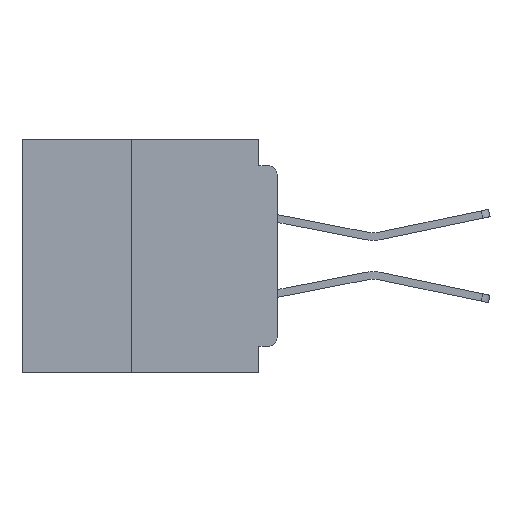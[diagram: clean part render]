
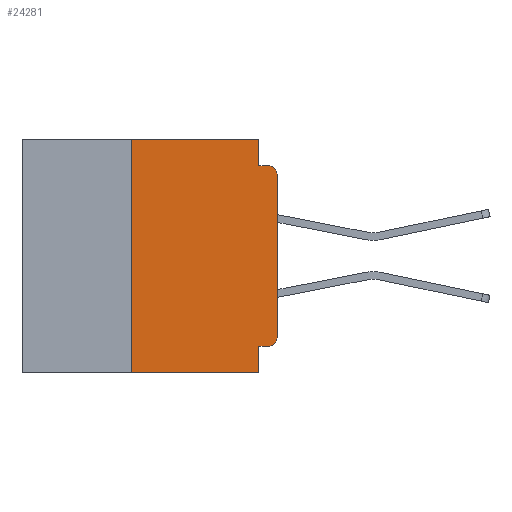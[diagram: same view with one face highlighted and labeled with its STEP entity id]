
A CAD part, left-side view. The second image highlights one B-rep face of the part: STEP entity #24281.
In plain terms, the highlighted planar face has unit normal (-1, 0, 0).
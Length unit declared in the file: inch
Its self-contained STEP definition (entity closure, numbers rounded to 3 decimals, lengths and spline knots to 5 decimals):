
#169 = EDGE_CURVE ( 'NONE', #33190, #14834, #8546, .T. ) ;
#683 = AXIS2_PLACEMENT_3D ( 'NONE', #11805, #33521, #14911 ) ;
#696 = LINE ( 'NONE', #1604, #8038 ) ;
#1527 = DIRECTION ( 'NONE',  ( 0., 0., -1. ) ) ;
#1538 = DIRECTION ( 'NONE',  ( 0., 0., -1. ) ) ;
#1604 = CARTESIAN_POINT ( 'NONE',  ( 0., 0., -0.045 ) ) ;
#1689 = AXIS2_PLACEMENT_3D ( 'NONE', #35556, #29384, #1527 ) ;
#1912 = CARTESIAN_POINT ( 'NONE',  ( 0., 0.031, -0.4 ) ) ;
#3444 = AXIS2_PLACEMENT_3D ( 'NONE', #34811, #16224, #37923 ) ;
#4148 = VERTEX_POINT ( 'NONE', #24754 ) ;
#4276 = VECTOR ( 'NONE', #1538, 39.37008 ) ;
#4750 = LINE ( 'NONE', #22648, #12005 ) ;
#5132 = CARTESIAN_POINT ( 'NONE',  ( 0., 0.031, -0.045 ) ) ;
#5250 = DIRECTION ( 'NONE',  ( 0., -1., 0. ) ) ;
#6891 = CARTESIAN_POINT ( 'NONE',  ( 0., 0.031, -0.355 ) ) ;
#6967 = VERTEX_POINT ( 'NONE', #36861 ) ;
#7402 = CARTESIAN_POINT ( 'NONE',  ( 0., 0.437, 0. ) ) ;
#7459 = EDGE_CURVE ( 'NONE', #32794, #4148, #23890, .T. ) ;
#7644 = CARTESIAN_POINT ( 'NONE',  ( 0., 0.031, 0. ) ) ;
#8038 = VECTOR ( 'NONE', #20191, 39.37008 ) ;
#8229 = ORIENTED_EDGE ( 'NONE', *, *, #169, .T. ) ;
#8308 = ORIENTED_EDGE ( 'NONE', *, *, #9075, .T. ) ;
#8374 = VECTOR ( 'NONE', #29146, 39.37008 ) ;
#8546 = LINE ( 'NONE', #17950, #32329 ) ;
#9075 = EDGE_CURVE ( 'NONE', #14834, #6967, #13033, .T. ) ;
#9210 = ORIENTED_EDGE ( 'NONE', *, *, #35574, .F. ) ;
#9241 = ORIENTED_EDGE ( 'NONE', *, *, #33174, .F. ) ;
#9282 = ORIENTED_EDGE ( 'NONE', *, *, #21765, .F. ) ;
#9529 = EDGE_CURVE ( 'NONE', #21045, #4148, #20307, .T. ) ;
#10096 = CARTESIAN_POINT ( 'NONE',  ( 0., 0.015, -0.355 ) ) ;
#10304 = ORIENTED_EDGE ( 'NONE', *, *, #37301, .F. ) ;
#10667 = ORIENTED_EDGE ( 'NONE', *, *, #7459, .T. ) ;
#10715 = VERTEX_POINT ( 'NONE', #35857 ) ;
#11273 = DIRECTION ( 'NONE',  ( 0., 0., -1. ) ) ;
#11653 = ORIENTED_EDGE ( 'NONE', *, *, #9529, .F. ) ;
#11805 = CARTESIAN_POINT ( 'NONE',  ( 0., 0.015, -0.34 ) ) ;
#12005 = VECTOR ( 'NONE', #25786, 39.37008 ) ;
#12025 = VECTOR ( 'NONE', #11273, 39.37008 ) ;
#12119 = ORIENTED_EDGE ( 'NONE', *, *, #38951, .F. ) ;
#12506 = LINE ( 'NONE', #7644, #4276 ) ;
#12916 = ORIENTED_EDGE ( 'NONE', *, *, #27837, .T. ) ;
#13033 = CIRCLE ( 'NONE', #3444, 0.015 ) ;
#13760 = VERTEX_POINT ( 'NONE', #5132 ) ;
#14834 = VERTEX_POINT ( 'NONE', #26094 ) ;
#14911 = DIRECTION ( 'NONE',  ( 0., 0., -1. ) ) ;
#15737 = LINE ( 'NONE', #18630, #16736 ) ;
#16224 = DIRECTION ( 'NONE',  ( -1., 0., 0. ) ) ;
#16736 = VECTOR ( 'NONE', #37328, 39.37008 ) ;
#17771 = CARTESIAN_POINT ( 'NONE',  ( 0., 0.031, 0. ) ) ;
#17950 = CARTESIAN_POINT ( 'NONE',  ( 0., 0., 0. ) ) ;
#18630 = CARTESIAN_POINT ( 'NONE',  ( 0., 0., -0.355 ) ) ;
#20112 = PLANE ( 'NONE',  #1689 ) ;
#20191 = DIRECTION ( 'NONE',  ( 0., -1., 0. ) ) ;
#20307 = LINE ( 'NONE', #1912, #12025 ) ;
#20724 = CARTESIAN_POINT ( 'NONE',  ( 0., 0.437, -0.4 ) ) ;
#21045 = VERTEX_POINT ( 'NONE', #6891 ) ;
#21765 = EDGE_CURVE ( 'NONE', #10715, #39937, #32151, .T. ) ;
#22648 = CARTESIAN_POINT ( 'NONE',  ( 0., 0.25, -0.4 ) ) ;
#23249 = EDGE_LOOP ( 'NONE', ( #8229, #8308, #9210, #9241, #9282, #10304, #10667, #11653, #12119, #12916 ) ) ;
#23252 = CARTESIAN_POINT ( 'NONE',  ( 0., 0., -0.34 ) ) ;
#23890 = LINE ( 'NONE', #20724, #31172 ) ;
#23947 = CARTESIAN_POINT ( 'NONE',  ( 0., 0.25, -0.4 ) ) ;
#24281 = ADVANCED_FACE ( 'NONE', ( #39240 ), #20112, .F. ) ;
#24754 = CARTESIAN_POINT ( 'NONE',  ( 0., 0.031, -0.4 ) ) ;
#25786 = DIRECTION ( 'NONE',  ( 0., 0., 1. ) ) ;
#26094 = CARTESIAN_POINT ( 'NONE',  ( 0., 0., -0.06 ) ) ;
#27492 = CIRCLE ( 'NONE', #683, 0.015 ) ;
#27837 = EDGE_CURVE ( 'NONE', #33033, #33190, #27492, .T. ) ;
#29146 = DIRECTION ( 'NONE',  ( 0., -1., 0. ) ) ;
#29384 = DIRECTION ( 'NONE',  ( 1., 0., 0. ) ) ;
#31172 = VECTOR ( 'NONE', #5250, 39.37008 ) ;
#32151 = LINE ( 'NONE', #7402, #8374 ) ;
#32329 = VECTOR ( 'NONE', #39949, 39.37008 ) ;
#32794 = VERTEX_POINT ( 'NONE', #23947 ) ;
#33033 = VERTEX_POINT ( 'NONE', #10096 ) ;
#33174 = EDGE_CURVE ( 'NONE', #39937, #13760, #12506, .T. ) ;
#33190 = VERTEX_POINT ( 'NONE', #23252 ) ;
#33521 = DIRECTION ( 'NONE',  ( -1., 0., 0. ) ) ;
#34811 = CARTESIAN_POINT ( 'NONE',  ( 0., 0.015, -0.06 ) ) ;
#35556 = CARTESIAN_POINT ( 'NONE',  ( 0., 0.437, 0. ) ) ;
#35574 = EDGE_CURVE ( 'NONE', #13760, #6967, #696, .T. ) ;
#35857 = CARTESIAN_POINT ( 'NONE',  ( 0., 0.25, 0. ) ) ;
#36861 = CARTESIAN_POINT ( 'NONE',  ( 0., 0.015, -0.045 ) ) ;
#37301 = EDGE_CURVE ( 'NONE', #32794, #10715, #4750, .T. ) ;
#37328 = DIRECTION ( 'NONE',  ( 0., 1., 0. ) ) ;
#37923 = DIRECTION ( 'NONE',  ( 0., 0., -1. ) ) ;
#38951 = EDGE_CURVE ( 'NONE', #33033, #21045, #15737, .T. ) ;
#39240 = FACE_OUTER_BOUND ( 'NONE', #23249, .T. ) ;
#39937 = VERTEX_POINT ( 'NONE', #17771 ) ;
#39949 = DIRECTION ( 'NONE',  ( 0., 0., 1. ) ) ;
